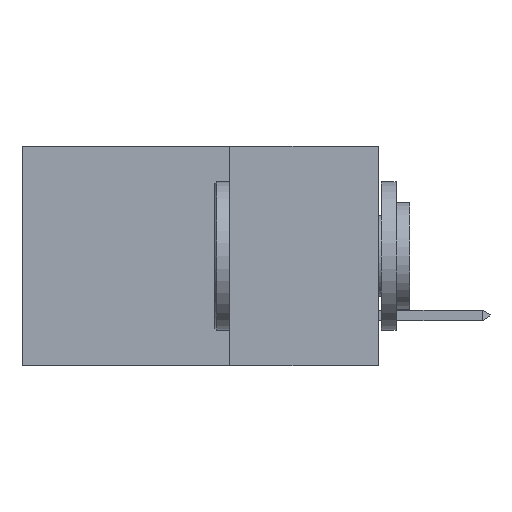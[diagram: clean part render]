
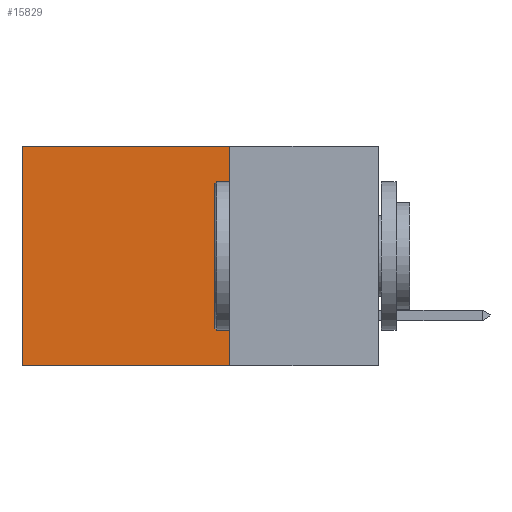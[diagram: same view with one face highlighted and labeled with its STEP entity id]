
A CAD part, left-side view. The second image highlights one B-rep face of the part: STEP entity #15829.
In plain terms, the highlighted planar face has unit normal (-1, 0, 0).
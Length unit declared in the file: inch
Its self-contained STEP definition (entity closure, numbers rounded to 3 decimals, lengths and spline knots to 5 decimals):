
#604 = CARTESIAN_POINT ( 'NONE',  ( 0.298, 0.25, 0. ) ) ;
#1284 = DIRECTION ( 'NONE',  ( 0., 1., 0. ) ) ;
#1735 = ORIENTED_EDGE ( 'NONE', *, *, #11158, .T. ) ;
#2128 = DIRECTION ( 'NONE',  ( 0., 0., -1. ) ) ;
#2208 = FACE_OUTER_BOUND ( 'NONE', #6192, .T. ) ;
#2980 = ORIENTED_EDGE ( 'NONE', *, *, #13753, .T. ) ;
#3118 = LINE ( 'NONE', #10130, #6518 ) ;
#3199 = VECTOR ( 'NONE', #21282, 39.37008 ) ;
#4569 = AXIS2_PLACEMENT_3D ( 'NONE', #10543, #15893, #17734 ) ;
#4698 = VECTOR ( 'NONE', #19513, 39.37008 ) ;
#6192 = EDGE_LOOP ( 'NONE', ( #2980, #14386, #21557, #1735 ) ) ;
#6518 = VECTOR ( 'NONE', #1284, 39.37008 ) ;
#8246 = CARTESIAN_POINT ( 'NONE',  ( 0.298, 0.6, 0. ) ) ;
#9489 = LINE ( 'NONE', #18028, #4698 ) ;
#10130 = CARTESIAN_POINT ( 'NONE',  ( 0.298, 0.25, -0.37 ) ) ;
#10543 = CARTESIAN_POINT ( 'NONE',  ( 0.298, 0.25, 0. ) ) ;
#10770 = PLANE ( 'NONE',  #4569 ) ;
#11158 = EDGE_CURVE ( 'NONE', #17534, #22556, #17310, .T. ) ;
#11430 = VERTEX_POINT ( 'NONE', #18470 ) ;
#12937 = EDGE_CURVE ( 'NONE', #17534, #11430, #22798, .T. ) ;
#13753 = EDGE_CURVE ( 'NONE', #22556, #18393, #9489, .T. ) ;
#14218 = CARTESIAN_POINT ( 'NONE',  ( 0.298, 0.25, 0. ) ) ;
#14386 = ORIENTED_EDGE ( 'NONE', *, *, #19292, .F. ) ;
#15829 = ADVANCED_FACE ( 'NONE', ( #2208 ), #10770, .F. ) ;
#15893 = DIRECTION ( 'NONE',  ( 1., 0., 0. ) ) ;
#16249 = CARTESIAN_POINT ( 'NONE',  ( 0.298, 0.6, -0.37 ) ) ;
#17310 = LINE ( 'NONE', #19773, #3199 ) ;
#17534 = VERTEX_POINT ( 'NONE', #14218 ) ;
#17734 = DIRECTION ( 'NONE',  ( 0., 0., -1. ) ) ;
#18020 = VECTOR ( 'NONE', #2128, 39.37008 ) ;
#18028 = CARTESIAN_POINT ( 'NONE',  ( 0.298, 0.6, 0. ) ) ;
#18393 = VERTEX_POINT ( 'NONE', #16249 ) ;
#18470 = CARTESIAN_POINT ( 'NONE',  ( 0.298, 0.25, -0.37 ) ) ;
#19292 = EDGE_CURVE ( 'NONE', #11430, #18393, #3118, .T. ) ;
#19513 = DIRECTION ( 'NONE',  ( 0., 0., -1. ) ) ;
#19773 = CARTESIAN_POINT ( 'NONE',  ( 0.298, 0.25, 0. ) ) ;
#21282 = DIRECTION ( 'NONE',  ( 0., 1., 0. ) ) ;
#21557 = ORIENTED_EDGE ( 'NONE', *, *, #12937, .F. ) ;
#22556 = VERTEX_POINT ( 'NONE', #8246 ) ;
#22798 = LINE ( 'NONE', #604, #18020 ) ;
